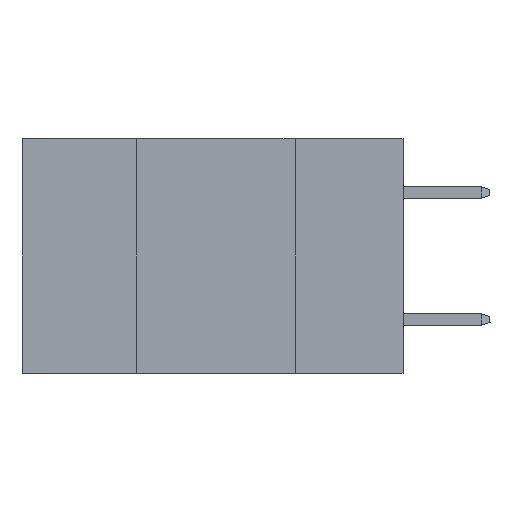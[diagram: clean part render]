
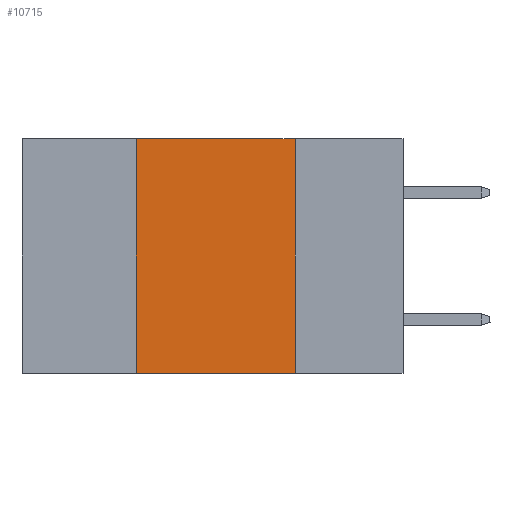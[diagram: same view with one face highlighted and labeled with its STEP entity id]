
A CAD part, left-side view. The second image highlights one B-rep face of the part: STEP entity #10715.
In plain terms, the highlighted planar face has unit normal (-1, 0, 0).
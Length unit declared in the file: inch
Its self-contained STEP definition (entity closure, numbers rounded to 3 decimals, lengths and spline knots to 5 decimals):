
#298 = CARTESIAN_POINT ( 'NONE',  ( 0., 0.42, 0. ) ) ;
#1251 = CARTESIAN_POINT ( 'NONE',  ( 0., 0.17, 0. ) ) ;
#3610 = EDGE_LOOP ( 'NONE', ( #17894, #6308, #5685, #10803 ) ) ;
#5685 = ORIENTED_EDGE ( 'NONE', *, *, #9971, .F. ) ;
#6308 = ORIENTED_EDGE ( 'NONE', *, *, #22618, .F. ) ;
#6999 = DIRECTION ( 'NONE',  ( 0., 0., -1. ) ) ;
#7100 = PLANE ( 'NONE',  #16261 ) ;
#7155 = VERTEX_POINT ( 'NONE', #7848 ) ;
#7848 = CARTESIAN_POINT ( 'NONE',  ( 0., 0.17, -0.37 ) ) ;
#9971 = EDGE_CURVE ( 'NONE', #23985, #20397, #12944, .T. ) ;
#10715 = ADVANCED_FACE ( 'NONE', ( #18374 ), #7100, .F. ) ;
#10803 = ORIENTED_EDGE ( 'NONE', *, *, #10820, .T. ) ;
#10820 = EDGE_CURVE ( 'NONE', #23985, #7155, #20400, .T. ) ;
#11748 = CARTESIAN_POINT ( 'NONE',  ( 0., 0.17, 0. ) ) ;
#11771 = DIRECTION ( 'NONE',  ( 0., -1., 0. ) ) ;
#12112 = EDGE_CURVE ( 'NONE', #13146, #7155, #13503, .T. ) ;
#12346 = LINE ( 'NONE', #13943, #27592 ) ;
#12944 = LINE ( 'NONE', #26530, #15300 ) ;
#13146 = VERTEX_POINT ( 'NONE', #1251 ) ;
#13503 = LINE ( 'NONE', #11748, #24131 ) ;
#13943 = CARTESIAN_POINT ( 'NONE',  ( 0., 0.6, 0. ) ) ;
#14308 = DIRECTION ( 'NONE',  ( 0., 0., -1. ) ) ;
#15300 = VECTOR ( 'NONE', #24930, 39.37008 ) ;
#16261 = AXIS2_PLACEMENT_3D ( 'NONE', #25146, #27173, #14308 ) ;
#17894 = ORIENTED_EDGE ( 'NONE', *, *, #12112, .F. ) ;
#18374 = FACE_OUTER_BOUND ( 'NONE', #3610, .T. ) ;
#18589 = VECTOR ( 'NONE', #18665, 39.37008 ) ;
#18665 = DIRECTION ( 'NONE',  ( 0., -1., 0. ) ) ;
#20397 = VERTEX_POINT ( 'NONE', #298 ) ;
#20400 = LINE ( 'NONE', #27035, #18589 ) ;
#22096 = CARTESIAN_POINT ( 'NONE',  ( 0., 0.42, -0.37 ) ) ;
#22618 = EDGE_CURVE ( 'NONE', #20397, #13146, #12346, .T. ) ;
#23985 = VERTEX_POINT ( 'NONE', #22096 ) ;
#24131 = VECTOR ( 'NONE', #6999, 39.37008 ) ;
#24930 = DIRECTION ( 'NONE',  ( 0., 0., 1. ) ) ;
#25146 = CARTESIAN_POINT ( 'NONE',  ( 0., 0.6, 0. ) ) ;
#26530 = CARTESIAN_POINT ( 'NONE',  ( 0., 0.42, 0. ) ) ;
#27035 = CARTESIAN_POINT ( 'NONE',  ( 0., 0.6, -0.37 ) ) ;
#27173 = DIRECTION ( 'NONE',  ( 1., 0., 0. ) ) ;
#27592 = VECTOR ( 'NONE', #11771, 39.37008 ) ;
